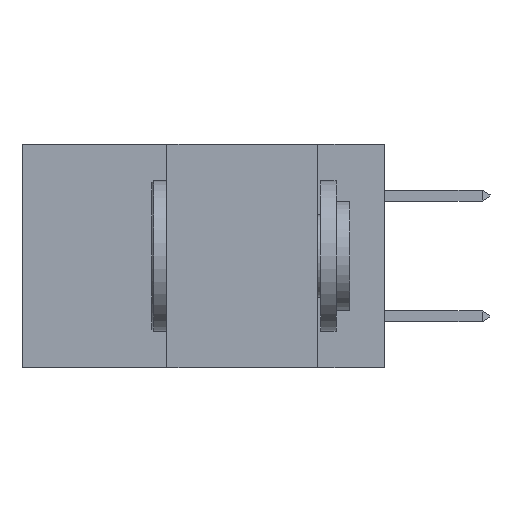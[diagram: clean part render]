
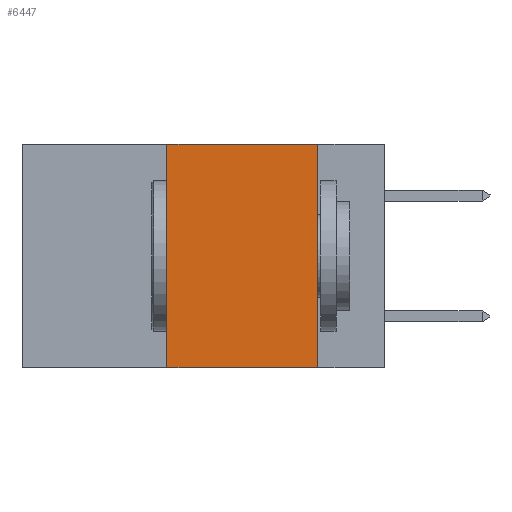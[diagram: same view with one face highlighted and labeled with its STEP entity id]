
A CAD part, left-side view. The second image highlights one B-rep face of the part: STEP entity #6447.
In plain terms, the highlighted planar face has unit normal (-1, 0, 0).
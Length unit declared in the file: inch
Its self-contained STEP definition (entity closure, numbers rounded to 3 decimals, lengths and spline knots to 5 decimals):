
#1433 = AXIS2_PLACEMENT_3D ( 'NONE', #11118, #23808, #13348 ) ;
#2433 = LINE ( 'NONE', #3532, #14069 ) ;
#3525 = EDGE_CURVE ( 'NONE', #19408, #4400, #2433, .T. ) ;
#3532 = CARTESIAN_POINT ( 'NONE',  ( 0., 0.6, -0.37 ) ) ;
#4400 = VERTEX_POINT ( 'NONE', #13428 ) ;
#4613 = VERTEX_POINT ( 'NONE', #27116 ) ;
#5625 = ORIENTED_EDGE ( 'NONE', *, *, #14627, .F. ) ;
#6250 = DIRECTION ( 'NONE',  ( 0., 0., -1. ) ) ;
#6447 = ADVANCED_FACE ( 'NONE', ( #17900 ), #21460, .F. ) ;
#6798 = LINE ( 'NONE', #15599, #22114 ) ;
#6879 = ORIENTED_EDGE ( 'NONE', *, *, #32264, .F. ) ;
#8101 = LINE ( 'NONE', #11656, #27807 ) ;
#8294 = CARTESIAN_POINT ( 'NONE',  ( 0., 0.36, -0.37 ) ) ;
#11118 = CARTESIAN_POINT ( 'NONE',  ( 0., 0.6, 0. ) ) ;
#11656 = CARTESIAN_POINT ( 'NONE',  ( 0., 0.11, 0. ) ) ;
#12586 = CARTESIAN_POINT ( 'NONE',  ( 0., 0.36, 0. ) ) ;
#12823 = VECTOR ( 'NONE', #25574, 39.37008 ) ;
#13348 = DIRECTION ( 'NONE',  ( 0., 0., -1. ) ) ;
#13428 = CARTESIAN_POINT ( 'NONE',  ( 0., 0.11, -0.37 ) ) ;
#14069 = VECTOR ( 'NONE', #28678, 39.37008 ) ;
#14627 = EDGE_CURVE ( 'NONE', #19408, #29825, #17622, .T. ) ;
#15599 = CARTESIAN_POINT ( 'NONE',  ( 0., 0.6, 0. ) ) ;
#15939 = DIRECTION ( 'NONE',  ( 0., -1., 0. ) ) ;
#17622 = LINE ( 'NONE', #12586, #12823 ) ;
#17900 = FACE_OUTER_BOUND ( 'NONE', #21799, .T. ) ;
#19408 = VERTEX_POINT ( 'NONE', #8294 ) ;
#21460 = PLANE ( 'NONE',  #1433 ) ;
#21799 = EDGE_LOOP ( 'NONE', ( #29222, #6879, #5625, #27600 ) ) ;
#22114 = VECTOR ( 'NONE', #15939, 39.37008 ) ;
#23808 = DIRECTION ( 'NONE',  ( 1., 0., 0. ) ) ;
#25463 = CARTESIAN_POINT ( 'NONE',  ( 0., 0.36, 0. ) ) ;
#25574 = DIRECTION ( 'NONE',  ( 0., 0., 1. ) ) ;
#27116 = CARTESIAN_POINT ( 'NONE',  ( 0., 0.11, 0. ) ) ;
#27600 = ORIENTED_EDGE ( 'NONE', *, *, #3525, .T. ) ;
#27807 = VECTOR ( 'NONE', #6250, 39.37008 ) ;
#28678 = DIRECTION ( 'NONE',  ( 0., -1., 0. ) ) ;
#29222 = ORIENTED_EDGE ( 'NONE', *, *, #30184, .F. ) ;
#29825 = VERTEX_POINT ( 'NONE', #25463 ) ;
#30184 = EDGE_CURVE ( 'NONE', #4613, #4400, #8101, .T. ) ;
#32264 = EDGE_CURVE ( 'NONE', #29825, #4613, #6798, .T. ) ;
